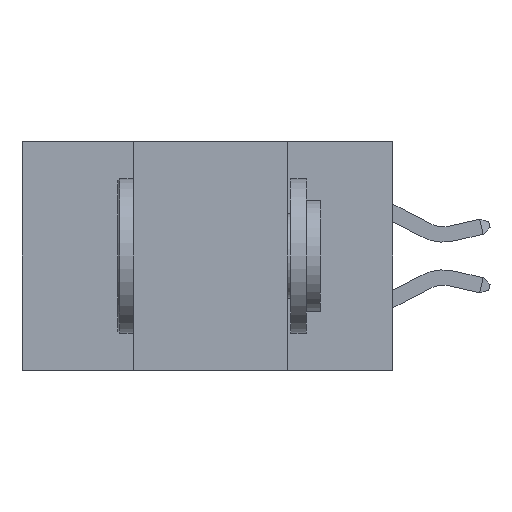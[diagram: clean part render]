
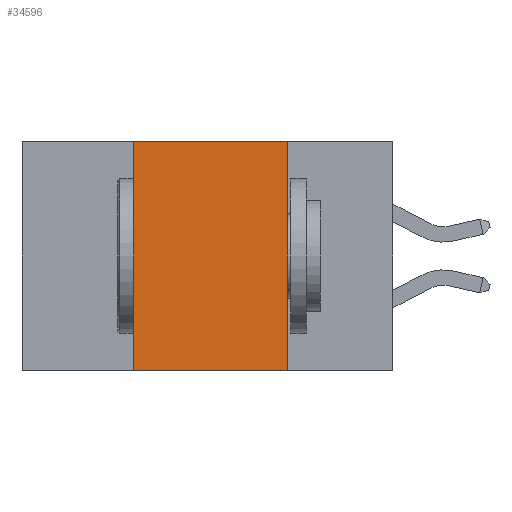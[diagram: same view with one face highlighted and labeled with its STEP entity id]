
A CAD part, left-side view. The second image highlights one B-rep face of the part: STEP entity #34596.
In plain terms, the highlighted planar face has unit normal (-1, 0, 0).
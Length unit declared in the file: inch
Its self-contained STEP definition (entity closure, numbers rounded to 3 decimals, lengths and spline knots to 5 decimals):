
#1543 = CARTESIAN_POINT ( 'NONE',  ( 0., 0.6, 0. ) ) ;
#2227 = LINE ( 'NONE', #14182, #31481 ) ;
#2951 = DIRECTION ( 'NONE',  ( 0., -1., 0. ) ) ;
#3800 = VERTEX_POINT ( 'NONE', #29507 ) ;
#4416 = PLANE ( 'NONE',  #8884 ) ;
#4474 = FACE_OUTER_BOUND ( 'NONE', #32688, .T. ) ;
#6677 = VERTEX_POINT ( 'NONE', #16500 ) ;
#7300 = DIRECTION ( 'NONE',  ( 0., 0., -1. ) ) ;
#8884 = AXIS2_PLACEMENT_3D ( 'NONE', #1543, #24260, #7300 ) ;
#9560 = VECTOR ( 'NONE', #2951, 39.37008 ) ;
#10438 = EDGE_CURVE ( 'NONE', #18613, #29487, #16164, .T. ) ;
#10443 = VECTOR ( 'NONE', #21094, 39.37008 ) ;
#12657 = CARTESIAN_POINT ( 'NONE',  ( 0., 0.17, 0. ) ) ;
#13376 = CARTESIAN_POINT ( 'NONE',  ( 0., 0.6, -0.37 ) ) ;
#14182 = CARTESIAN_POINT ( 'NONE',  ( 0., 0.42, 0. ) ) ;
#15726 = EDGE_CURVE ( 'NONE', #6677, #3800, #36134, .T. ) ;
#16164 = LINE ( 'NONE', #19944, #9560 ) ;
#16500 = CARTESIAN_POINT ( 'NONE',  ( 0., 0.42, -0.37 ) ) ;
#18296 = ORIENTED_EDGE ( 'NONE', *, *, #10438, .F. ) ;
#18613 = VERTEX_POINT ( 'NONE', #19910 ) ;
#19910 = CARTESIAN_POINT ( 'NONE',  ( 0., 0.42, 0. ) ) ;
#19944 = CARTESIAN_POINT ( 'NONE',  ( 0., 0.6, 0. ) ) ;
#20074 = ORIENTED_EDGE ( 'NONE', *, *, #23338, .F. ) ;
#20251 = EDGE_CURVE ( 'NONE', #29487, #3800, #26413, .T. ) ;
#21094 = DIRECTION ( 'NONE',  ( 0., 0., -1. ) ) ;
#22098 = VECTOR ( 'NONE', #30338, 39.37008 ) ;
#22729 = DIRECTION ( 'NONE',  ( 0., 0., 1. ) ) ;
#23338 = EDGE_CURVE ( 'NONE', #6677, #18613, #2227, .T. ) ;
#24056 = ORIENTED_EDGE ( 'NONE', *, *, #20251, .F. ) ;
#24260 = DIRECTION ( 'NONE',  ( 1., 0., 0. ) ) ;
#26413 = LINE ( 'NONE', #32298, #10443 ) ;
#29399 = ORIENTED_EDGE ( 'NONE', *, *, #15726, .T. ) ;
#29487 = VERTEX_POINT ( 'NONE', #12657 ) ;
#29507 = CARTESIAN_POINT ( 'NONE',  ( 0., 0.17, -0.37 ) ) ;
#30338 = DIRECTION ( 'NONE',  ( 0., -1., 0. ) ) ;
#31481 = VECTOR ( 'NONE', #22729, 39.37008 ) ;
#32298 = CARTESIAN_POINT ( 'NONE',  ( 0., 0.17, 0. ) ) ;
#32688 = EDGE_LOOP ( 'NONE', ( #24056, #18296, #20074, #29399 ) ) ;
#34596 = ADVANCED_FACE ( 'NONE', ( #4474 ), #4416, .F. ) ;
#36134 = LINE ( 'NONE', #13376, #22098 ) ;
